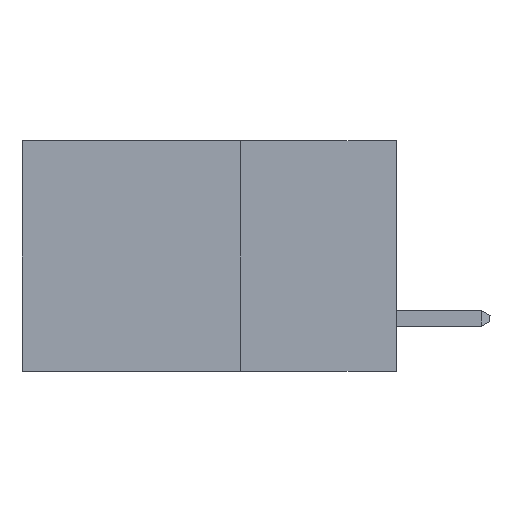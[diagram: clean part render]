
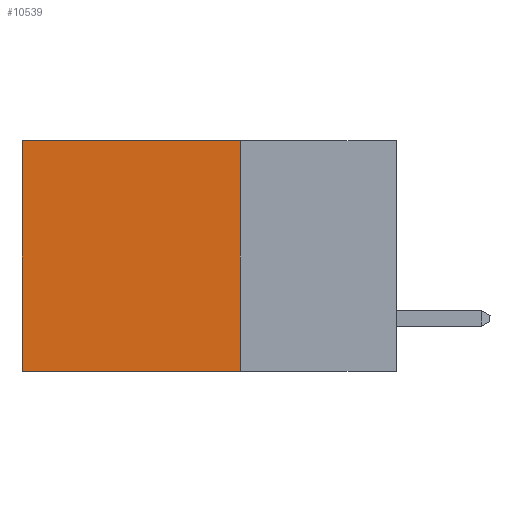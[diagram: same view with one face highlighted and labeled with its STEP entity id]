
A CAD part, left-side view. The second image highlights one B-rep face of the part: STEP entity #10539.
In plain terms, the highlighted planar face has unit normal (-1, 0, 0).
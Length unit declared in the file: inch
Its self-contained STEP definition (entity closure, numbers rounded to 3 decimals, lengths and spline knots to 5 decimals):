
#557 = ORIENTED_EDGE ( 'NONE', *, *, #5371, .T. ) ;
#614 = DIRECTION ( 'NONE',  ( 0., 1., 0. ) ) ;
#695 = VECTOR ( 'NONE', #10211, 39.37008 ) ;
#1202 = CARTESIAN_POINT ( 'NONE',  ( 0.2615, 0.25, 0. ) ) ;
#1297 = LINE ( 'NONE', #1487, #6364 ) ;
#1448 = CARTESIAN_POINT ( 'NONE',  ( 0.2615, 0.6, 0. ) ) ;
#1487 = CARTESIAN_POINT ( 'NONE',  ( 0.2615, 0.25, -0.37 ) ) ;
#1952 = ORIENTED_EDGE ( 'NONE', *, *, #5698, .F. ) ;
#2080 = ORIENTED_EDGE ( 'NONE', *, *, #9716, .T. ) ;
#2184 = CARTESIAN_POINT ( 'NONE',  ( 0.2615, 0.25, 0. ) ) ;
#2568 = VERTEX_POINT ( 'NONE', #6034 ) ;
#3504 = LINE ( 'NONE', #8767, #11478 ) ;
#4638 = VECTOR ( 'NONE', #10424, 39.37008 ) ;
#4984 = PLANE ( 'NONE',  #5470 ) ;
#5371 = EDGE_CURVE ( 'NONE', #5406, #2568, #9763, .T. ) ;
#5406 = VERTEX_POINT ( 'NONE', #1448 ) ;
#5470 = AXIS2_PLACEMENT_3D ( 'NONE', #10397, #6940, #7711 ) ;
#5698 = EDGE_CURVE ( 'NONE', #9316, #10364, #1297, .T. ) ;
#5971 = LINE ( 'NONE', #1202, #695 ) ;
#6034 = CARTESIAN_POINT ( 'NONE',  ( 0.2615, 0.6, -0.37 ) ) ;
#6136 = EDGE_LOOP ( 'NONE', ( #557, #7752, #1952, #2080 ) ) ;
#6364 = VECTOR ( 'NONE', #6829, 39.37008 ) ;
#6701 = FACE_OUTER_BOUND ( 'NONE', #6136, .T. ) ;
#6829 = DIRECTION ( 'NONE',  ( 0., 0., -1. ) ) ;
#6940 = DIRECTION ( 'NONE',  ( 1., 0., 0. ) ) ;
#7711 = DIRECTION ( 'NONE',  ( 0., 0., -1. ) ) ;
#7752 = ORIENTED_EDGE ( 'NONE', *, *, #9945, .F. ) ;
#8767 = CARTESIAN_POINT ( 'NONE',  ( 0.2615, 0.25, -0.37 ) ) ;
#9316 = VERTEX_POINT ( 'NONE', #2184 ) ;
#9716 = EDGE_CURVE ( 'NONE', #9316, #5406, #5971, .T. ) ;
#9763 = LINE ( 'NONE', #11387, #4638 ) ;
#9945 = EDGE_CURVE ( 'NONE', #10364, #2568, #3504, .T. ) ;
#10211 = DIRECTION ( 'NONE',  ( 0., 1., 0. ) ) ;
#10364 = VERTEX_POINT ( 'NONE', #11445 ) ;
#10397 = CARTESIAN_POINT ( 'NONE',  ( 0.2615, 0.25, -0.37 ) ) ;
#10424 = DIRECTION ( 'NONE',  ( 0., 0., -1. ) ) ;
#10539 = ADVANCED_FACE ( 'NONE', ( #6701 ), #4984, .F. ) ;
#11387 = CARTESIAN_POINT ( 'NONE',  ( 0.2615, 0.6, -0.37 ) ) ;
#11445 = CARTESIAN_POINT ( 'NONE',  ( 0.2615, 0.25, -0.37 ) ) ;
#11478 = VECTOR ( 'NONE', #614, 39.37008 ) ;
